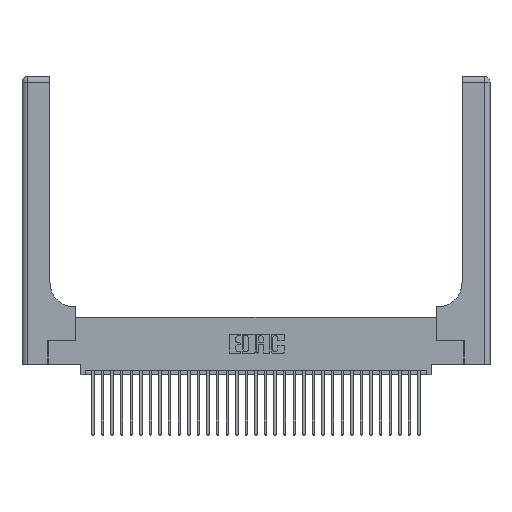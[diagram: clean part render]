
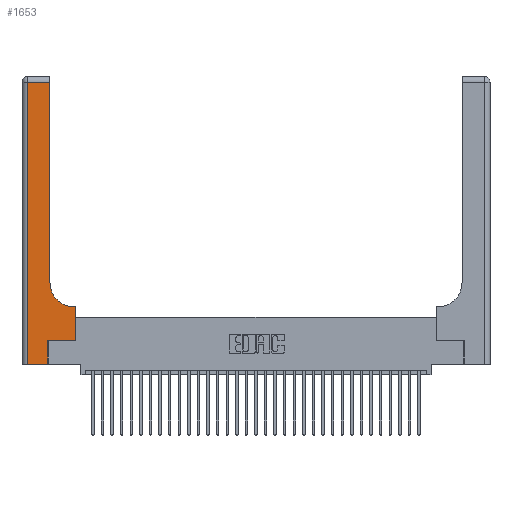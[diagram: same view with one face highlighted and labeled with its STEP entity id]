
A CAD part, top view. The second image highlights one B-rep face of the part: STEP entity #1653.
In plain terms, the highlighted planar face has unit normal (0, 0, 1).
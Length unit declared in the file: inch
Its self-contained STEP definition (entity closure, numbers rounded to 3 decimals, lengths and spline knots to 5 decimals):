
#31 = DIRECTION ( 'NONE',  ( 0., 0., -1. ) ) ;
#678 = VERTEX_POINT ( 'NONE', #32744 ) ;
#825 = CARTESIAN_POINT ( 'NONE',  ( 0.269, 0.25, 0.37 ) ) ;
#1200 = EDGE_CURVE ( 'NONE', #26698, #23421, #20162, .T. ) ;
#1314 = ORIENTED_EDGE ( 'NONE', *, *, #22942, .T. ) ;
#1642 = VECTOR ( 'NONE', #22914, 39.37008 ) ;
#1653 = ADVANCED_FACE ( 'NONE', ( #17242 ), #20531, .F. ) ;
#1820 = EDGE_CURVE ( 'NONE', #24245, #18174, #16032, .T. ) ;
#2126 = ORIENTED_EDGE ( 'NONE', *, *, #1820, .T. ) ;
#2200 = CARTESIAN_POINT ( 'NONE',  ( 0.2915, 3., 0.37 ) ) ;
#2372 = CARTESIAN_POINT ( 'NONE',  ( 0.5415, 0.85, 0.37 ) ) ;
#3244 = EDGE_LOOP ( 'NONE', ( #9150, #10868, #31388, #1314, #11221, #25790, #25887, #32681, #2126 ) ) ;
#3945 = VERTEX_POINT ( 'NONE', #13295 ) ;
#4088 = VECTOR ( 'NONE', #18802, 39.37008 ) ;
#4723 = DIRECTION ( 'NONE',  ( 1., 0., 0. ) ) ;
#6814 = EDGE_CURVE ( 'NONE', #10245, #678, #16920, .T. ) ;
#7123 = VECTOR ( 'NONE', #7562, 39.37008 ) ;
#7562 = DIRECTION ( 'NONE',  ( 0., 1., 0. ) ) ;
#8865 = LINE ( 'NONE', #13169, #17449 ) ;
#9150 = ORIENTED_EDGE ( 'NONE', *, *, #11749, .T. ) ;
#9676 = VECTOR ( 'NONE', #17123, 39.37008 ) ;
#10245 = VERTEX_POINT ( 'NONE', #825 ) ;
#10868 = ORIENTED_EDGE ( 'NONE', *, *, #33611, .T. ) ;
#11221 = ORIENTED_EDGE ( 'NONE', *, *, #25337, .T. ) ;
#11563 = VECTOR ( 'NONE', #33093, 39.37008 ) ;
#11749 = EDGE_CURVE ( 'NONE', #18174, #20770, #14046, .T. ) ;
#13169 = CARTESIAN_POINT ( 'NONE',  ( 0.269, 0., 0.37 ) ) ;
#13295 = CARTESIAN_POINT ( 'NONE',  ( 0.269, 0., 0.37 ) ) ;
#14046 = LINE ( 'NONE', #2200, #7123 ) ;
#14083 = VECTOR ( 'NONE', #4723, 39.37008 ) ;
#14175 = LINE ( 'NONE', #25101, #9676 ) ;
#14221 = VERTEX_POINT ( 'NONE', #30695 ) ;
#15482 = CARTESIAN_POINT ( 'NONE',  ( 0.06, 0., 0.37 ) ) ;
#15625 = CARTESIAN_POINT ( 'NONE',  ( 0., 3., 0.37 ) ) ;
#16032 = CIRCLE ( 'NONE', #16966, 0.25 ) ;
#16247 = LINE ( 'NONE', #18818, #25646 ) ;
#16421 = CARTESIAN_POINT ( 'NONE',  ( 0.5415, 0.6, 0.37 ) ) ;
#16920 = LINE ( 'NONE', #29220, #14083 ) ;
#16932 = EDGE_CURVE ( 'NONE', #14221, #24245, #24060, .T. ) ;
#16966 = AXIS2_PLACEMENT_3D ( 'NONE', #2372, #33426, #20391 ) ;
#17123 = DIRECTION ( 'NONE',  ( -1., 0., 0. ) ) ;
#17242 = FACE_OUTER_BOUND ( 'NONE', #3244, .T. ) ;
#17449 = VECTOR ( 'NONE', #29134, 39.37008 ) ;
#17975 = EDGE_CURVE ( 'NONE', #678, #14221, #16247, .T. ) ;
#18174 = VERTEX_POINT ( 'NONE', #30845 ) ;
#18802 = DIRECTION ( 'NONE',  ( 1., 0., 0. ) ) ;
#18818 = CARTESIAN_POINT ( 'NONE',  ( 0.5585, 0.25, 0.37 ) ) ;
#20162 = LINE ( 'NONE', #30448, #11563 ) ;
#20391 = DIRECTION ( 'NONE',  ( 1., 0., 0. ) ) ;
#20531 = PLANE ( 'NONE',  #28558 ) ;
#20770 = VERTEX_POINT ( 'NONE', #31580 ) ;
#22914 = DIRECTION ( 'NONE',  ( -1., 0., 0. ) ) ;
#22942 = EDGE_CURVE ( 'NONE', #23421, #3945, #24065, .T. ) ;
#23421 = VERTEX_POINT ( 'NONE', #15482 ) ;
#24060 = LINE ( 'NONE', #27959, #1642 ) ;
#24065 = LINE ( 'NONE', #29196, #4088 ) ;
#24245 = VERTEX_POINT ( 'NONE', #16421 ) ;
#25101 = CARTESIAN_POINT ( 'NONE',  ( 0., 2.94, 0.37 ) ) ;
#25337 = EDGE_CURVE ( 'NONE', #3945, #10245, #8865, .T. ) ;
#25646 = VECTOR ( 'NONE', #31962, 39.37008 ) ;
#25758 = DIRECTION ( 'NONE',  ( -1., 0., 0. ) ) ;
#25790 = ORIENTED_EDGE ( 'NONE', *, *, #6814, .T. ) ;
#25887 = ORIENTED_EDGE ( 'NONE', *, *, #17975, .T. ) ;
#26698 = VERTEX_POINT ( 'NONE', #32846 ) ;
#27959 = CARTESIAN_POINT ( 'NONE',  ( 0.2915, 0.6, 0.37 ) ) ;
#28558 = AXIS2_PLACEMENT_3D ( 'NONE', #15625, #31, #25758 ) ;
#29134 = DIRECTION ( 'NONE',  ( 0., 1., 0. ) ) ;
#29196 = CARTESIAN_POINT ( 'NONE',  ( 0., 0., 0.37 ) ) ;
#29220 = CARTESIAN_POINT ( 'NONE',  ( 0.269, 0.25, 0.37 ) ) ;
#30448 = CARTESIAN_POINT ( 'NONE',  ( 0.06, 3., 0.37 ) ) ;
#30695 = CARTESIAN_POINT ( 'NONE',  ( 0.5585, 0.6, 0.37 ) ) ;
#30845 = CARTESIAN_POINT ( 'NONE',  ( 0.2915, 0.85, 0.37 ) ) ;
#31388 = ORIENTED_EDGE ( 'NONE', *, *, #1200, .T. ) ;
#31580 = CARTESIAN_POINT ( 'NONE',  ( 0.2915, 2.94, 0.37 ) ) ;
#31962 = DIRECTION ( 'NONE',  ( 0., 1., 0. ) ) ;
#32681 = ORIENTED_EDGE ( 'NONE', *, *, #16932, .T. ) ;
#32744 = CARTESIAN_POINT ( 'NONE',  ( 0.5585, 0.25, 0.37 ) ) ;
#32846 = CARTESIAN_POINT ( 'NONE',  ( 0.06, 2.94, 0.37 ) ) ;
#33093 = DIRECTION ( 'NONE',  ( 0., -1., 0. ) ) ;
#33426 = DIRECTION ( 'NONE',  ( 0., 0., -1. ) ) ;
#33611 = EDGE_CURVE ( 'NONE', #20770, #26698, #14175, .T. ) ;
